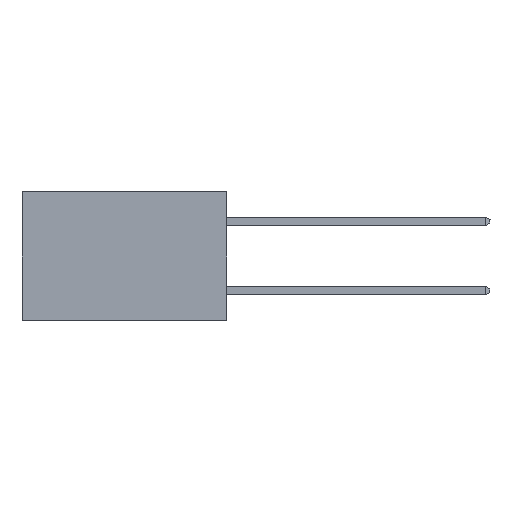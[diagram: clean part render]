
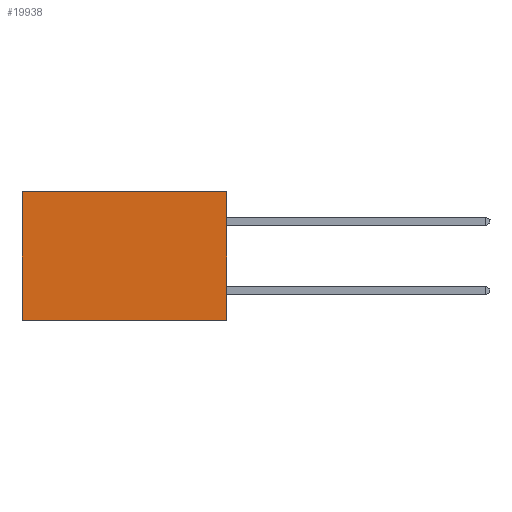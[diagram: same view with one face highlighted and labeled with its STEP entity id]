
A CAD part, left-side view. The second image highlights one B-rep face of the part: STEP entity #19938.
In plain terms, the highlighted planar face has unit normal (-1, 0, 0).
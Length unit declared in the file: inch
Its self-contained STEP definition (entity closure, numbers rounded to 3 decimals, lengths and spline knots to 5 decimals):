
#1257 = CARTESIAN_POINT ( 'NONE',  ( 0.277, 0., -0.37 ) ) ;
#1736 = VERTEX_POINT ( 'NONE', #14810 ) ;
#2170 = PLANE ( 'NONE',  #15050 ) ;
#3233 = CARTESIAN_POINT ( 'NONE',  ( 0.277, 0.59, -0.37 ) ) ;
#3262 = VERTEX_POINT ( 'NONE', #7729 ) ;
#3684 = LINE ( 'NONE', #21439, #7972 ) ;
#4057 = CARTESIAN_POINT ( 'NONE',  ( 0.277, 0., -0.37 ) ) ;
#4320 = CARTESIAN_POINT ( 'NONE',  ( 0.277, 0.59, 0. ) ) ;
#5934 = DIRECTION ( 'NONE',  ( 1., 0., 0. ) ) ;
#6187 = EDGE_CURVE ( 'NONE', #7119, #1736, #3684, .T. ) ;
#6314 = LINE ( 'NONE', #8355, #9918 ) ;
#6938 = DIRECTION ( 'NONE',  ( 0., 0., -1. ) ) ;
#7119 = VERTEX_POINT ( 'NONE', #1257 ) ;
#7729 = CARTESIAN_POINT ( 'NONE',  ( 0.277, 0., 0. ) ) ;
#7972 = VECTOR ( 'NONE', #21344, 39.37008 ) ;
#8050 = ORIENTED_EDGE ( 'NONE', *, *, #17283, .T. ) ;
#8355 = CARTESIAN_POINT ( 'NONE',  ( 0.277, 0., 0. ) ) ;
#8370 = EDGE_CURVE ( 'NONE', #19287, #1736, #11217, .T. ) ;
#8398 = CARTESIAN_POINT ( 'NONE',  ( 0.277, 0., -0.37 ) ) ;
#8890 = EDGE_LOOP ( 'NONE', ( #15204, #17747, #20402, #8050 ) ) ;
#9918 = VECTOR ( 'NONE', #11898, 39.37008 ) ;
#11217 = LINE ( 'NONE', #3233, #19970 ) ;
#11898 = DIRECTION ( 'NONE',  ( 0., 1., 0. ) ) ;
#12891 = VECTOR ( 'NONE', #20656, 39.37008 ) ;
#14810 = CARTESIAN_POINT ( 'NONE',  ( 0.277, 0.59, -0.37 ) ) ;
#15050 = AXIS2_PLACEMENT_3D ( 'NONE', #4057, #5934, #18283 ) ;
#15204 = ORIENTED_EDGE ( 'NONE', *, *, #8370, .T. ) ;
#17029 = LINE ( 'NONE', #8398, #12891 ) ;
#17283 = EDGE_CURVE ( 'NONE', #3262, #19287, #6314, .T. ) ;
#17747 = ORIENTED_EDGE ( 'NONE', *, *, #6187, .F. ) ;
#17780 = FACE_OUTER_BOUND ( 'NONE', #8890, .T. ) ;
#18283 = DIRECTION ( 'NONE',  ( 0., 0., -1. ) ) ;
#18761 = EDGE_CURVE ( 'NONE', #3262, #7119, #17029, .T. ) ;
#19287 = VERTEX_POINT ( 'NONE', #4320 ) ;
#19938 = ADVANCED_FACE ( 'NONE', ( #17780 ), #2170, .F. ) ;
#19970 = VECTOR ( 'NONE', #6938, 39.37008 ) ;
#20402 = ORIENTED_EDGE ( 'NONE', *, *, #18761, .F. ) ;
#20656 = DIRECTION ( 'NONE',  ( 0., 0., -1. ) ) ;
#21344 = DIRECTION ( 'NONE',  ( 0., 1., 0. ) ) ;
#21439 = CARTESIAN_POINT ( 'NONE',  ( 0.277, 0., -0.37 ) ) ;
